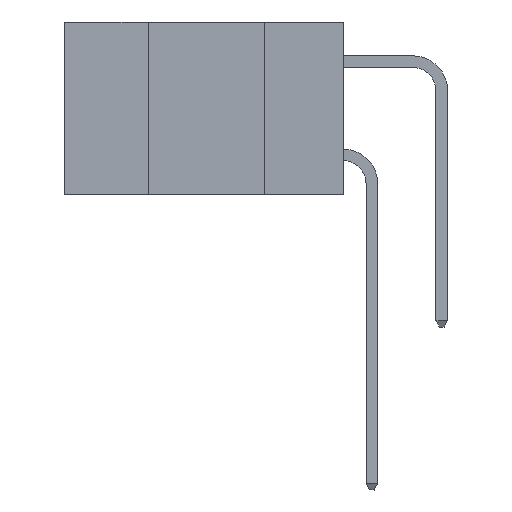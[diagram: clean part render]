
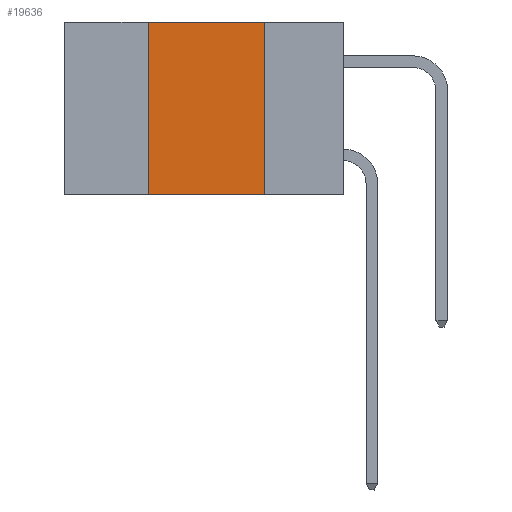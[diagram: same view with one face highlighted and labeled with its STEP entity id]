
A CAD part, left-side view. The second image highlights one B-rep face of the part: STEP entity #19636.
In plain terms, the highlighted planar face has unit normal (-1, 0, 0).
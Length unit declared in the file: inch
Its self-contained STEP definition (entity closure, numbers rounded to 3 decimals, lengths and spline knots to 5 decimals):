
#303 = EDGE_LOOP ( 'NONE', ( #33000, #19779, #10984, #25532 ) ) ;
#445 = DIRECTION ( 'NONE',  ( 0., 0., 1. ) ) ;
#1632 = CARTESIAN_POINT ( 'NONE',  ( 0., 0.17, 0. ) ) ;
#6412 = EDGE_CURVE ( 'NONE', #12983, #6527, #15222, .T. ) ;
#6527 = VERTEX_POINT ( 'NONE', #26108 ) ;
#7383 = CARTESIAN_POINT ( 'NONE',  ( 0., 0.17, 0. ) ) ;
#8121 = DIRECTION ( 'NONE',  ( 1., 0., 0. ) ) ;
#10984 = ORIENTED_EDGE ( 'NONE', *, *, #6412, .F. ) ;
#11283 = VERTEX_POINT ( 'NONE', #22823 ) ;
#11648 = EDGE_CURVE ( 'NONE', #30636, #11283, #26732, .T. ) ;
#12767 = CARTESIAN_POINT ( 'NONE',  ( 0., 0.42, 0. ) ) ;
#12983 = VERTEX_POINT ( 'NONE', #34403 ) ;
#13106 = VECTOR ( 'NONE', #19173, 39.37008 ) ;
#13596 = EDGE_CURVE ( 'NONE', #6527, #30636, #23023, .T. ) ;
#14395 = VECTOR ( 'NONE', #445, 39.37008 ) ;
#15222 = LINE ( 'NONE', #12767, #14395 ) ;
#18163 = EDGE_CURVE ( 'NONE', #12983, #11283, #20216, .T. ) ;
#18949 = PLANE ( 'NONE',  #24193 ) ;
#19173 = DIRECTION ( 'NONE',  ( 0., -1., 0. ) ) ;
#19636 = ADVANCED_FACE ( 'NONE', ( #23562 ), #18949, .F. ) ;
#19779 = ORIENTED_EDGE ( 'NONE', *, *, #13596, .F. ) ;
#20216 = LINE ( 'NONE', #27224, #13106 ) ;
#20289 = DIRECTION ( 'NONE',  ( 0., -1., 0. ) ) ;
#22823 = CARTESIAN_POINT ( 'NONE',  ( 0., 0.17, -0.37 ) ) ;
#23023 = LINE ( 'NONE', #33660, #30180 ) ;
#23378 = DIRECTION ( 'NONE',  ( 0., 0., -1. ) ) ;
#23562 = FACE_OUTER_BOUND ( 'NONE', #303, .T. ) ;
#24193 = AXIS2_PLACEMENT_3D ( 'NONE', #27002, #8121, #27118 ) ;
#25532 = ORIENTED_EDGE ( 'NONE', *, *, #18163, .T. ) ;
#25873 = VECTOR ( 'NONE', #23378, 39.37008 ) ;
#26108 = CARTESIAN_POINT ( 'NONE',  ( 0., 0.42, 0. ) ) ;
#26732 = LINE ( 'NONE', #1632, #25873 ) ;
#27002 = CARTESIAN_POINT ( 'NONE',  ( 0., 0.6, 0. ) ) ;
#27118 = DIRECTION ( 'NONE',  ( 0., 0., -1. ) ) ;
#27224 = CARTESIAN_POINT ( 'NONE',  ( 0., 0.6, -0.37 ) ) ;
#30180 = VECTOR ( 'NONE', #20289, 39.37008 ) ;
#30636 = VERTEX_POINT ( 'NONE', #7383 ) ;
#33000 = ORIENTED_EDGE ( 'NONE', *, *, #11648, .F. ) ;
#33660 = CARTESIAN_POINT ( 'NONE',  ( 0., 0.6, 0. ) ) ;
#34403 = CARTESIAN_POINT ( 'NONE',  ( 0., 0.42, -0.37 ) ) ;
